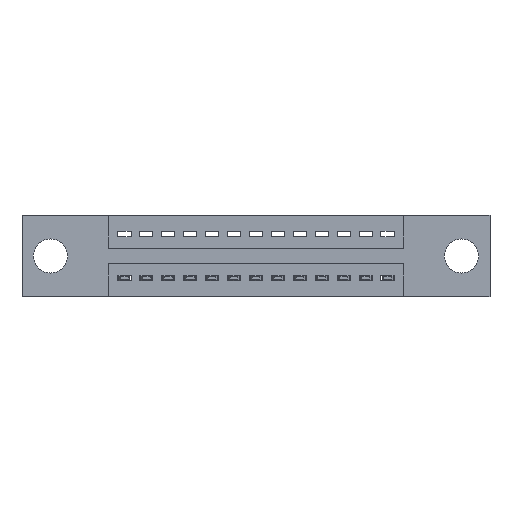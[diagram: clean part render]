
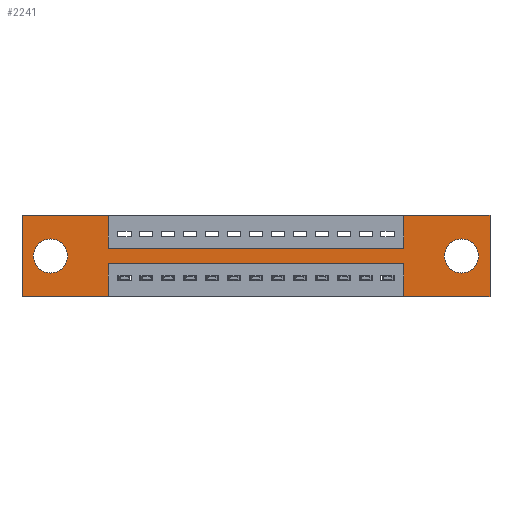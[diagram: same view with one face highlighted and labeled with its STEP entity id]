
A CAD part, front view. The second image highlights one B-rep face of the part: STEP entity #2241.
In plain terms, the highlighted planar face has unit normal (0, -1, 0).
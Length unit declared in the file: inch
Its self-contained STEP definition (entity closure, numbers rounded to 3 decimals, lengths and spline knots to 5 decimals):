
#57 = VERTEX_POINT ( 'NONE', #8275 ) ;
#118 = FACE_BOUND ( 'NONE', #1405, .T. ) ;
#252 = VERTEX_POINT ( 'NONE', #12525 ) ;
#405 = CIRCLE ( 'NONE', #13442, 0.078 ) ;
#456 = LINE ( 'NONE', #3012, #3438 ) ;
#535 = CARTESIAN_POINT ( 'NONE',  ( 0.3925, 0., -0.15 ) ) ;
#640 = FACE_BOUND ( 'NONE', #9935, .T. ) ;
#761 = CARTESIAN_POINT ( 'NONE',  ( 1.7425, 0., 0. ) ) ;
#991 = EDGE_CURVE ( 'NONE', #9303, #11129, #5579, .T. ) ;
#1031 = VERTEX_POINT ( 'NONE', #13141 ) ;
#1052 = VERTEX_POINT ( 'NONE', #7202 ) ;
#1375 = DIRECTION ( 'NONE',  ( 0., 1., 0. ) ) ;
#1405 = EDGE_LOOP ( 'NONE', ( #9751, #4090 ) ) ;
#1422 = ORIENTED_EDGE ( 'NONE', *, *, #7112, .F. ) ;
#1482 = VECTOR ( 'NONE', #7164, 39.37008 ) ;
#1570 = CARTESIAN_POINT ( 'NONE',  ( 0.3925, 0., -0.37 ) ) ;
#1603 = DIRECTION ( 'NONE',  ( 0., 0., 1. ) ) ;
#1868 = VECTOR ( 'NONE', #7199, 39.37008 ) ;
#2109 = EDGE_CURVE ( 'NONE', #8819, #12064, #3118, .T. ) ;
#2179 = EDGE_CURVE ( 'NONE', #12064, #10534, #456, .T. ) ;
#2229 = ORIENTED_EDGE ( 'NONE', *, *, #2109, .F. ) ;
#2241 = ADVANCED_FACE ( 'NONE', ( #640, #118, #12845 ), #10109, .T. ) ;
#2361 = ORIENTED_EDGE ( 'NONE', *, *, #4298, .F. ) ;
#2441 = CARTESIAN_POINT ( 'NONE',  ( 0.13, 0., -0.185 ) ) ;
#2582 = ORIENTED_EDGE ( 'NONE', *, *, #2179, .F. ) ;
#2777 = CARTESIAN_POINT ( 'NONE',  ( 2.135, 0., -0.37 ) ) ;
#2948 = VECTOR ( 'NONE', #10873, 39.37008 ) ;
#2966 = VECTOR ( 'NONE', #11644, 39.37008 ) ;
#3012 = CARTESIAN_POINT ( 'NONE',  ( 1.7425, 0., -0.37 ) ) ;
#3118 = LINE ( 'NONE', #12908, #2948 ) ;
#3140 = CIRCLE ( 'NONE', #11810, 0.078 ) ;
#3347 = VERTEX_POINT ( 'NONE', #4980 ) ;
#3438 = VECTOR ( 'NONE', #6145, 39.37008 ) ;
#3559 = CARTESIAN_POINT ( 'NONE',  ( 0.3925, 0., -0.22 ) ) ;
#3629 = ORIENTED_EDGE ( 'NONE', *, *, #5907, .F. ) ;
#3734 = DIRECTION ( 'NONE',  ( -1., 0., 0. ) ) ;
#3770 = LINE ( 'NONE', #8745, #9440 ) ;
#3837 = DIRECTION ( 'NONE',  ( -1., 0., 0. ) ) ;
#3943 = DIRECTION ( 'NONE',  ( 0., 0., -1. ) ) ;
#4027 = AXIS2_PLACEMENT_3D ( 'NONE', #7680, #1375, #10843 ) ;
#4045 = DIRECTION ( 'NONE',  ( 0., 0., 1. ) ) ;
#4090 = ORIENTED_EDGE ( 'NONE', *, *, #7464, .T. ) ;
#4163 = EDGE_CURVE ( 'NONE', #8248, #1052, #405, .T. ) ;
#4298 = EDGE_CURVE ( 'NONE', #57, #9303, #10519, .T. ) ;
#4542 = VECTOR ( 'NONE', #11155, 39.37008 ) ;
#4769 = VECTOR ( 'NONE', #4045, 39.37008 ) ;
#4952 = CARTESIAN_POINT ( 'NONE',  ( 2.005, 0., -0.185 ) ) ;
#4967 = VERTEX_POINT ( 'NONE', #535 ) ;
#4980 = CARTESIAN_POINT ( 'NONE',  ( 0.13, 0., -0.263 ) ) ;
#5094 = LINE ( 'NONE', #1570, #8653 ) ;
#5242 = VECTOR ( 'NONE', #3734, 39.37008 ) ;
#5361 = VERTEX_POINT ( 'NONE', #6014 ) ;
#5400 = EDGE_CURVE ( 'NONE', #4967, #11306, #10991, .T. ) ;
#5579 = LINE ( 'NONE', #8438, #10146 ) ;
#5750 = LINE ( 'NONE', #11121, #1482 ) ;
#5878 = DIRECTION ( 'NONE',  ( 1., 0., 0. ) ) ;
#5907 = EDGE_CURVE ( 'NONE', #252, #6598, #8538, .T. ) ;
#5927 = AXIS2_PLACEMENT_3D ( 'NONE', #6868, #8851, #1603 ) ;
#6014 = CARTESIAN_POINT ( 'NONE',  ( 0.3925, 0., -0.37 ) ) ;
#6145 = DIRECTION ( 'NONE',  ( 0., 0., 1. ) ) ;
#6171 = CIRCLE ( 'NONE', #5927, 0.078 ) ;
#6288 = ORIENTED_EDGE ( 'NONE', *, *, #9616, .T. ) ;
#6351 = CARTESIAN_POINT ( 'NONE',  ( 1.7425, 0., -0.22 ) ) ;
#6510 = DIRECTION ( 'NONE',  ( 0., 0., 1. ) ) ;
#6598 = VERTEX_POINT ( 'NONE', #8294 ) ;
#6780 = DIRECTION ( 'NONE',  ( 0., 0., -1. ) ) ;
#6868 = CARTESIAN_POINT ( 'NONE',  ( 0.13, 0., -0.185 ) ) ;
#6975 = CARTESIAN_POINT ( 'NONE',  ( 0., 0., 0. ) ) ;
#7112 = EDGE_CURVE ( 'NONE', #11129, #4967, #5750, .T. ) ;
#7164 = DIRECTION ( 'NONE',  ( 0., 0., -1. ) ) ;
#7199 = DIRECTION ( 'NONE',  ( 1., 0., 0. ) ) ;
#7202 = CARTESIAN_POINT ( 'NONE',  ( 2.005, 0., -0.107 ) ) ;
#7402 = CARTESIAN_POINT ( 'NONE',  ( 1.7425, 0., -0.15 ) ) ;
#7422 = CARTESIAN_POINT ( 'NONE',  ( 0.3925, 0., 0. ) ) ;
#7432 = DIRECTION ( 'NONE',  ( 1., 0., 0. ) ) ;
#7464 = EDGE_CURVE ( 'NONE', #3347, #1031, #3140, .T. ) ;
#7511 = LINE ( 'NONE', #761, #4769 ) ;
#7589 = EDGE_CURVE ( 'NONE', #9540, #5361, #5094, .T. ) ;
#7680 = CARTESIAN_POINT ( 'NONE',  ( 2.005, 0., -0.185 ) ) ;
#8015 = EDGE_CURVE ( 'NONE', #11306, #252, #7511, .T. ) ;
#8156 = LINE ( 'NONE', #10497, #2966 ) ;
#8248 = VERTEX_POINT ( 'NONE', #10303 ) ;
#8275 = CARTESIAN_POINT ( 'NONE',  ( 0., 0., -0.37 ) ) ;
#8294 = CARTESIAN_POINT ( 'NONE',  ( 2.135, 0., 0. ) ) ;
#8438 = CARTESIAN_POINT ( 'NONE',  ( 0., 0., 0. ) ) ;
#8538 = LINE ( 'NONE', #12938, #8860 ) ;
#8653 = VECTOR ( 'NONE', #6780, 39.37008 ) ;
#8745 = CARTESIAN_POINT ( 'NONE',  ( 0., 0., -0.37 ) ) ;
#8819 = VERTEX_POINT ( 'NONE', #2777 ) ;
#8851 = DIRECTION ( 'NONE',  ( 0., 1., 0. ) ) ;
#8860 = VECTOR ( 'NONE', #5878, 39.37008 ) ;
#9303 = VERTEX_POINT ( 'NONE', #12463 ) ;
#9388 = EDGE_CURVE ( 'NONE', #1031, #3347, #6171, .T. ) ;
#9440 = VECTOR ( 'NONE', #3837, 39.37008 ) ;
#9460 = LINE ( 'NONE', #10839, #5242 ) ;
#9470 = CIRCLE ( 'NONE', #4027, 0.078 ) ;
#9540 = VERTEX_POINT ( 'NONE', #3559 ) ;
#9616 = EDGE_CURVE ( 'NONE', #1052, #8248, #9470, .T. ) ;
#9711 = EDGE_LOOP ( 'NONE', ( #9775, #9858, #2582, #2229, #11451, #3629, #11050, #11816, #1422, #13166, #2361, #12963 ) ) ;
#9751 = ORIENTED_EDGE ( 'NONE', *, *, #9388, .T. ) ;
#9775 = ORIENTED_EDGE ( 'NONE', *, *, #7589, .F. ) ;
#9858 = ORIENTED_EDGE ( 'NONE', *, *, #10034, .F. ) ;
#9935 = EDGE_LOOP ( 'NONE', ( #6288, #10779 ) ) ;
#10034 = EDGE_CURVE ( 'NONE', #10534, #9540, #9460, .T. ) ;
#10097 = AXIS2_PLACEMENT_3D ( 'NONE', #10148, #11200, #11253 ) ;
#10109 = PLANE ( 'NONE',  #10097 ) ;
#10146 = VECTOR ( 'NONE', #7432, 39.37008 ) ;
#10148 = CARTESIAN_POINT ( 'NONE',  ( 0., 0., -0.37 ) ) ;
#10162 = DIRECTION ( 'NONE',  ( 0., 1., 0. ) ) ;
#10303 = CARTESIAN_POINT ( 'NONE',  ( 2.005, 0., -0.263 ) ) ;
#10497 = CARTESIAN_POINT ( 'NONE',  ( 2.135, 0., 0. ) ) ;
#10519 = LINE ( 'NONE', #6975, #4542 ) ;
#10534 = VERTEX_POINT ( 'NONE', #6351 ) ;
#10617 = EDGE_CURVE ( 'NONE', #5361, #57, #3770, .T. ) ;
#10779 = ORIENTED_EDGE ( 'NONE', *, *, #4163, .T. ) ;
#10839 = CARTESIAN_POINT ( 'NONE',  ( 0.3925, 0., -0.22 ) ) ;
#10843 = DIRECTION ( 'NONE',  ( 0., 0., -1. ) ) ;
#10873 = DIRECTION ( 'NONE',  ( -1., 0., 0. ) ) ;
#10933 = EDGE_CURVE ( 'NONE', #6598, #8819, #8156, .T. ) ;
#10991 = LINE ( 'NONE', #11377, #1868 ) ;
#11050 = ORIENTED_EDGE ( 'NONE', *, *, #8015, .F. ) ;
#11121 = CARTESIAN_POINT ( 'NONE',  ( 0.3925, 0., 0. ) ) ;
#11129 = VERTEX_POINT ( 'NONE', #7422 ) ;
#11155 = DIRECTION ( 'NONE',  ( 0., 0., 1. ) ) ;
#11200 = DIRECTION ( 'NONE',  ( 0., -1., 0. ) ) ;
#11253 = DIRECTION ( 'NONE',  ( 0., 0., -1. ) ) ;
#11306 = VERTEX_POINT ( 'NONE', #7402 ) ;
#11377 = CARTESIAN_POINT ( 'NONE',  ( 0.3925, 0., -0.15 ) ) ;
#11451 = ORIENTED_EDGE ( 'NONE', *, *, #10933, .F. ) ;
#11594 = CARTESIAN_POINT ( 'NONE',  ( 1.7425, 0., -0.37 ) ) ;
#11644 = DIRECTION ( 'NONE',  ( 0., 0., -1. ) ) ;
#11810 = AXIS2_PLACEMENT_3D ( 'NONE', #2441, #12718, #6510 ) ;
#11816 = ORIENTED_EDGE ( 'NONE', *, *, #5400, .F. ) ;
#12064 = VERTEX_POINT ( 'NONE', #11594 ) ;
#12463 = CARTESIAN_POINT ( 'NONE',  ( 0., 0., 0. ) ) ;
#12525 = CARTESIAN_POINT ( 'NONE',  ( 1.7425, 0., 0. ) ) ;
#12718 = DIRECTION ( 'NONE',  ( 0., 1., 0. ) ) ;
#12845 = FACE_OUTER_BOUND ( 'NONE', #9711, .T. ) ;
#12908 = CARTESIAN_POINT ( 'NONE',  ( 0., 0., -0.37 ) ) ;
#12938 = CARTESIAN_POINT ( 'NONE',  ( 0., 0., 0. ) ) ;
#12963 = ORIENTED_EDGE ( 'NONE', *, *, #10617, .F. ) ;
#13141 = CARTESIAN_POINT ( 'NONE',  ( 0.13, 0., -0.107 ) ) ;
#13166 = ORIENTED_EDGE ( 'NONE', *, *, #991, .F. ) ;
#13442 = AXIS2_PLACEMENT_3D ( 'NONE', #4952, #10162, #3943 ) ;
